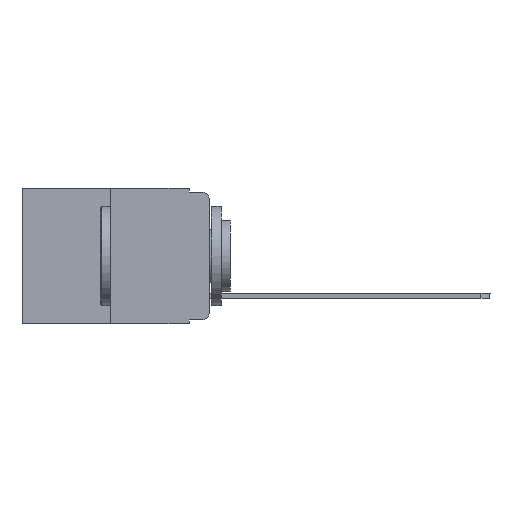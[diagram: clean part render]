
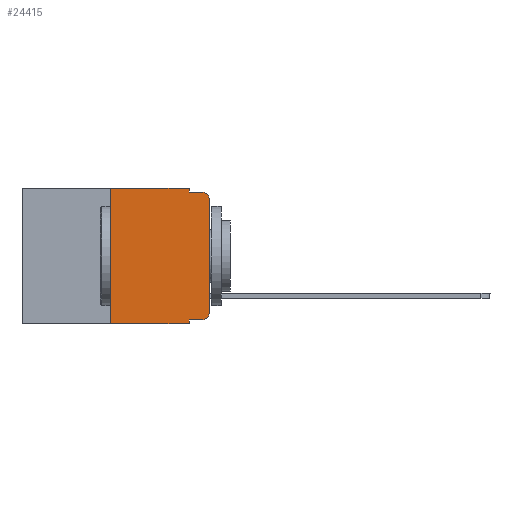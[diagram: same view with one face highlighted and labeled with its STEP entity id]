
A CAD part, left-side view. The second image highlights one B-rep face of the part: STEP entity #24415.
In plain terms, the highlighted planar face has unit normal (-1, 0, 0).
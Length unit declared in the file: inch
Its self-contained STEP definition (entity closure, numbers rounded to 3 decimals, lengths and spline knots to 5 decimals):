
#45 = DIRECTION ( 'NONE',  ( 0., 0., -1. ) ) ;
#228 = CARTESIAN_POINT ( 'NONE',  ( 0., 0.051, -0.01 ) ) ;
#694 = VECTOR ( 'NONE', #7739, 39.37008 ) ;
#713 = VERTEX_POINT ( 'NONE', #10699 ) ;
#750 = CARTESIAN_POINT ( 'NONE',  ( 0., 0.051, 0. ) ) ;
#817 = VERTEX_POINT ( 'NONE', #24402 ) ;
#1140 = DIRECTION ( 'NONE',  ( 0., 0., -1. ) ) ;
#2178 = VECTOR ( 'NONE', #11092, 39.37008 ) ;
#2283 = DIRECTION ( 'NONE',  ( 0., 0., -1. ) ) ;
#2814 = DIRECTION ( 'NONE',  ( 0., 0., -1. ) ) ;
#3085 = LINE ( 'NONE', #15576, #2178 ) ;
#3436 = VERTEX_POINT ( 'NONE', #3481 ) ;
#3481 = CARTESIAN_POINT ( 'NONE',  ( 0., 0.25, 0. ) ) ;
#4796 = PLANE ( 'NONE',  #23156 ) ;
#4841 = EDGE_CURVE ( 'NONE', #19439, #3436, #24252, .T. ) ;
#5711 = DIRECTION ( 'NONE',  ( 0., 0., 1. ) ) ;
#6217 = CARTESIAN_POINT ( 'NONE',  ( 0., 0.25, 0. ) ) ;
#6294 = ORIENTED_EDGE ( 'NONE', *, *, #14076, .F. ) ;
#6310 = DIRECTION ( 'NONE',  ( 0., -1., 0. ) ) ;
#6687 = LINE ( 'NONE', #20245, #13541 ) ;
#6722 = EDGE_CURVE ( 'NONE', #7894, #11763, #22719, .T. ) ;
#7720 = DIRECTION ( 'NONE',  ( -1., 0., 0. ) ) ;
#7739 = DIRECTION ( 'NONE',  ( 0., 0., 1. ) ) ;
#7894 = VERTEX_POINT ( 'NONE', #15230 ) ;
#8015 = ORIENTED_EDGE ( 'NONE', *, *, #20064, .T. ) ;
#8111 = CIRCLE ( 'NONE', #24502, 0.02 ) ;
#8274 = VECTOR ( 'NONE', #2283, 39.37008 ) ;
#8356 = CARTESIAN_POINT ( 'NONE',  ( 0., 0.02, -0.313 ) ) ;
#8487 = FACE_OUTER_BOUND ( 'NONE', #9774, .T. ) ;
#8658 = EDGE_CURVE ( 'NONE', #13997, #817, #8111, .T. ) ;
#8914 = VECTOR ( 'NONE', #24853, 39.37008 ) ;
#9223 = EDGE_CURVE ( 'NONE', #3436, #7894, #6687, .T. ) ;
#9281 = EDGE_CURVE ( 'NONE', #19439, #713, #19171, .T. ) ;
#9550 = ORIENTED_EDGE ( 'NONE', *, *, #23127, .T. ) ;
#9745 = ORIENTED_EDGE ( 'NONE', *, *, #6722, .F. ) ;
#9774 = EDGE_LOOP ( 'NONE', ( #8015, #9550, #23899, #9745, #22844, #10139, #19751, #6294, #14117, #23417 ) ) ;
#10139 = ORIENTED_EDGE ( 'NONE', *, *, #4841, .F. ) ;
#10260 = VERTEX_POINT ( 'NONE', #11494 ) ;
#10575 = DIRECTION ( 'NONE',  ( 1., 0., 0. ) ) ;
#10699 = CARTESIAN_POINT ( 'NONE',  ( 0., 0.051, -0.343 ) ) ;
#10960 = CARTESIAN_POINT ( 'NONE',  ( 0., 0.02, -0.01 ) ) ;
#11056 = VECTOR ( 'NONE', #5711, 39.37008 ) ;
#11092 = DIRECTION ( 'NONE',  ( 0., -1., 0. ) ) ;
#11364 = CIRCLE ( 'NONE', #19332, 0.02 ) ;
#11494 = CARTESIAN_POINT ( 'NONE',  ( 0., 0., -0.03 ) ) ;
#11763 = VERTEX_POINT ( 'NONE', #228 ) ;
#11897 = CARTESIAN_POINT ( 'NONE',  ( 0., 0.02, -0.333 ) ) ;
#12061 = LINE ( 'NONE', #25766, #694 ) ;
#12816 = CARTESIAN_POINT ( 'NONE',  ( 0., 0.473, 0. ) ) ;
#12997 = VECTOR ( 'NONE', #1140, 39.37008 ) ;
#13541 = VECTOR ( 'NONE', #18388, 39.37008 ) ;
#13997 = VERTEX_POINT ( 'NONE', #11897 ) ;
#14076 = EDGE_CURVE ( 'NONE', #14502, #713, #20551, .T. ) ;
#14117 = ORIENTED_EDGE ( 'NONE', *, *, #24605, .T. ) ;
#14502 = VERTEX_POINT ( 'NONE', #18276 ) ;
#15230 = CARTESIAN_POINT ( 'NONE',  ( 0., 0.051, 0. ) ) ;
#15576 = CARTESIAN_POINT ( 'NONE',  ( 0., 0.051, -0.333 ) ) ;
#16241 = VERTEX_POINT ( 'NONE', #10960 ) ;
#16811 = CARTESIAN_POINT ( 'NONE',  ( 0., 0.473, -0.343 ) ) ;
#18276 = CARTESIAN_POINT ( 'NONE',  ( 0., 0.051, -0.333 ) ) ;
#18283 = EDGE_CURVE ( 'NONE', #11763, #16241, #22489, .T. ) ;
#18309 = CARTESIAN_POINT ( 'NONE',  ( 0., 0.051, 0. ) ) ;
#18388 = DIRECTION ( 'NONE',  ( 0., -1., 0. ) ) ;
#19171 = LINE ( 'NONE', #16811, #8914 ) ;
#19332 = AXIS2_PLACEMENT_3D ( 'NONE', #25743, #7720, #23757 ) ;
#19439 = VERTEX_POINT ( 'NONE', #25263 ) ;
#19751 = ORIENTED_EDGE ( 'NONE', *, *, #9281, .T. ) ;
#20064 = EDGE_CURVE ( 'NONE', #817, #10260, #12061, .T. ) ;
#20245 = CARTESIAN_POINT ( 'NONE',  ( 0., 0.473, 0. ) ) ;
#20309 = DIRECTION ( 'NONE',  ( -1., 0., 0. ) ) ;
#20551 = LINE ( 'NONE', #18309, #8274 ) ;
#20553 = VECTOR ( 'NONE', #6310, 39.37008 ) ;
#22489 = LINE ( 'NONE', #24352, #20553 ) ;
#22719 = LINE ( 'NONE', #750, #12997 ) ;
#22844 = ORIENTED_EDGE ( 'NONE', *, *, #9223, .F. ) ;
#23127 = EDGE_CURVE ( 'NONE', #10260, #16241, #11364, .T. ) ;
#23156 = AXIS2_PLACEMENT_3D ( 'NONE', #12816, #10575, #2814 ) ;
#23417 = ORIENTED_EDGE ( 'NONE', *, *, #8658, .T. ) ;
#23757 = DIRECTION ( 'NONE',  ( 0., 0., -1. ) ) ;
#23899 = ORIENTED_EDGE ( 'NONE', *, *, #18283, .F. ) ;
#24252 = LINE ( 'NONE', #6217, #11056 ) ;
#24352 = CARTESIAN_POINT ( 'NONE',  ( 0., 0.051, -0.01 ) ) ;
#24402 = CARTESIAN_POINT ( 'NONE',  ( 0., 0., -0.313 ) ) ;
#24415 = ADVANCED_FACE ( 'NONE', ( #8487 ), #4796, .F. ) ;
#24502 = AXIS2_PLACEMENT_3D ( 'NONE', #8356, #20309, #45 ) ;
#24605 = EDGE_CURVE ( 'NONE', #14502, #13997, #3085, .T. ) ;
#24853 = DIRECTION ( 'NONE',  ( 0., -1., 0. ) ) ;
#25263 = CARTESIAN_POINT ( 'NONE',  ( 0., 0.25, -0.343 ) ) ;
#25743 = CARTESIAN_POINT ( 'NONE',  ( 0., 0.02, -0.03 ) ) ;
#25766 = CARTESIAN_POINT ( 'NONE',  ( 0., 0., 0. ) ) ;
